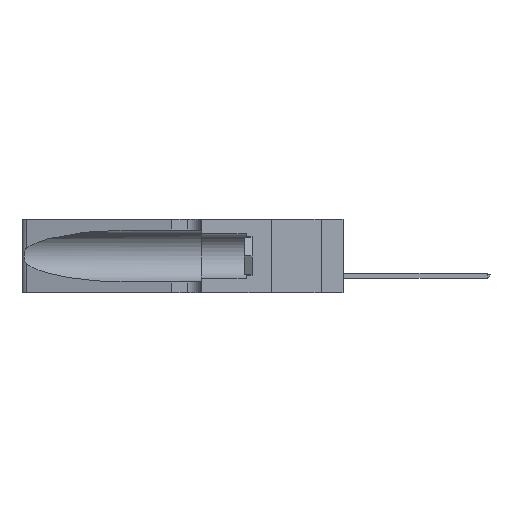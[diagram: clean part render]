
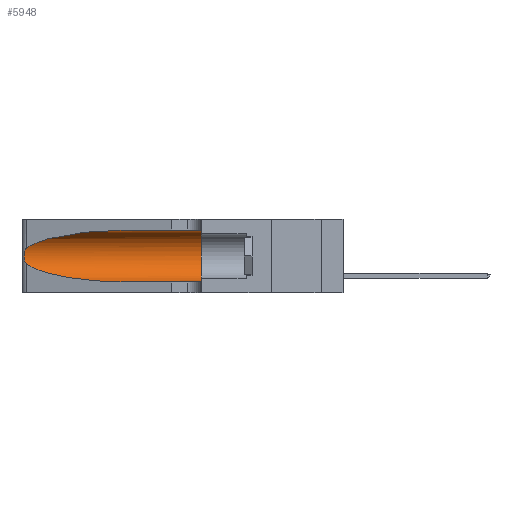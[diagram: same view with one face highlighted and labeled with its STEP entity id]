
A CAD part, left-side view. The second image highlights one B-rep face of the part: STEP entity #5948.
In plain terms, the highlighted cylindrical face has radius 3.308 mm (diameter 6.617 mm), a partial arc.
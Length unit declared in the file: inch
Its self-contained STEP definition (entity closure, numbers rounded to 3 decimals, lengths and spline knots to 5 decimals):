
#655 = CARTESIAN_POINT ( 'NONE',  ( 0.25555, 1.22993, 0.14849 ) ) ;
#1748 = LINE ( 'NONE', #39697, #17648 ) ;
#3922 = ORIENTED_EDGE ( 'NONE', *, *, #5991, .F. ) ;
#4035 = VECTOR ( 'NONE', #27838, 39.37008 ) ;
#4862 = CARTESIAN_POINT ( 'NONE',  ( 0.1305, 1.61858, 0.05475 ) ) ;
#5517 = EDGE_CURVE ( 'NONE', #15986, #20509, #34708, .T. ) ;
#5948 = ADVANCED_FACE ( 'NONE', ( #23339 ), #35680, .F. ) ;
#5991 = EDGE_CURVE ( 'NONE', #20962, #15986, #1748, .T. ) ;
#6048 = CARTESIAN_POINT ( 'NONE',  ( 0.1305, 0.35, 0.185 ) ) ;
#6563 = CARTESIAN_POINT ( 'NONE',  ( 0.26018, 1.23835, 0.19895 ) ) ;
#6578 = VERTEX_POINT ( 'NONE', #8494 ) ;
#6843 = CARTESIAN_POINT ( 'NONE',  ( 0.25487, 1.22718, 0.14631 ) ) ;
#7131 = CARTESIAN_POINT ( 'NONE',  ( 0.25639, 1.23186, 0.15144 ) ) ;
#7521 = AXIS2_PLACEMENT_3D ( 'NONE', #28760, #9085, #19129 ) ;
#8494 = CARTESIAN_POINT ( 'NONE',  ( 0.25487, 1.22718, 0.22369 ) ) ;
#9085 = DIRECTION ( 'NONE',  ( 0., -1., 0. ) ) ;
#9271 = CARTESIAN_POINT ( 'NONE',  ( 0.26075, 1.23896, 0.19203 ) ) ;
#9691 = CARTESIAN_POINT ( 'NONE',  ( 0.25789, 1.23486, 0.15765 ) ) ;
#9707 = VERTEX_POINT ( 'NONE', #18508 ) ;
#10004 = CARTESIAN_POINT ( 'NONE',  ( 0.1305, 0.72297, 0.31525 ) ) ;
#10328 = EDGE_CURVE ( 'NONE', #6578, #23851, #29841, .T. ) ;
#11489 = ORIENTED_EDGE ( 'NONE', *, *, #18581, .T. ) ;
#11865 = CARTESIAN_POINT ( 'NONE',  ( 0.18966, 0.96281, 0.05475 ) ) ;
#13286 = CARTESIAN_POINT ( 'NONE',  ( 0.18966, 0.96281, 0.31525 ) ) ;
#14525 =( BOUNDED_CURVE ( )  B_SPLINE_CURVE ( 3, ( #10004, #13286, #26381, #36300 ),
 .UNSPECIFIED., .F., .T. ) 
 B_SPLINE_CURVE_WITH_KNOTS ( ( 4, 4 ),
 ( 1.5708, 2.84003 ),
 .UNSPECIFIED. ) 
 CURVE ( )  GEOMETRIC_REPRESENTATION_ITEM ( )  RATIONAL_B_SPLINE_CURVE ( ( 1., 0.87, 0.87, 1. ) ) 
 REPRESENTATION_ITEM ( '' )  );
#15850 = CARTESIAN_POINT ( 'NONE',  ( 0.26075, 1.23896, 0.178 ) ) ;
#15986 = VERTEX_POINT ( 'NONE', #32086 ) ;
#17013 = ORIENTED_EDGE ( 'NONE', *, *, #5517, .F. ) ;
#17648 = VECTOR ( 'NONE', #29626, 39.37008 ) ;
#18508 = CARTESIAN_POINT ( 'NONE',  ( 0.1305, 0.72297, 0.05475 ) ) ;
#18581 = EDGE_CURVE ( 'NONE', #9707, #20509, #19427, .T. ) ;
#18585 = CARTESIAN_POINT ( 'NONE',  ( 0.25487, 1.22718, 0.22369 ) ) ;
#18779 = CARTESIAN_POINT ( 'NONE',  ( 0.1305, 0.35, 0.05475 ) ) ;
#19129 = DIRECTION ( 'NONE',  ( 0., 0., -1. ) ) ;
#19427 = LINE ( 'NONE', #4862, #4035 ) ;
#20509 = VERTEX_POINT ( 'NONE', #18779 ) ;
#20924 = ORIENTED_EDGE ( 'NONE', *, *, #25940, .T. ) ;
#20962 = VERTEX_POINT ( 'NONE', #34828 ) ;
#22037 = CARTESIAN_POINT ( 'NONE',  ( 0.25787, 1.23484, 0.2124 ) ) ;
#22477 = CARTESIAN_POINT ( 'NONE',  ( 0.26017, 1.23833, 0.17102 ) ) ;
#22758 = CARTESIAN_POINT ( 'NONE',  ( 0.25856, 1.23593, 0.16098 ) ) ;
#23339 = FACE_OUTER_BOUND ( 'NONE', #27698, .T. ) ;
#23851 = VERTEX_POINT ( 'NONE', #37448 ) ;
#25346 = CARTESIAN_POINT ( 'NONE',  ( 0.25854, 1.2359, 0.20912 ) ) ;
#25940 = EDGE_CURVE ( 'NONE', #23851, #9707, #38251, .T. ) ;
#26177 = EDGE_CURVE ( 'NONE', #20962, #6578, #14525, .T. ) ;
#26381 = CARTESIAN_POINT ( 'NONE',  ( 0.2373, 1.15595, 0.28018 ) ) ;
#26403 = DIRECTION ( 'NONE',  ( 0., 0., 1. ) ) ;
#26969 = DIRECTION ( 'NONE',  ( 0., 1., 0. ) ) ;
#27698 = EDGE_LOOP ( 'NONE', ( #40674, #36368, #20924, #11489, #17013, #3922 ) ) ;
#27838 = DIRECTION ( 'NONE',  ( 0., -1., 0. ) ) ;
#28095 = CARTESIAN_POINT ( 'NONE',  ( 0.25487, 1.22718, 0.14631 ) ) ;
#28219 = CARTESIAN_POINT ( 'NONE',  ( 0.25555, 1.22994, 0.2215 ) ) ;
#28760 = CARTESIAN_POINT ( 'NONE',  ( 0.1305, 1.61858, 0.185 ) ) ;
#29626 = DIRECTION ( 'NONE',  ( 0., -1., 0. ) ) ;
#29841 = B_SPLINE_CURVE_WITH_KNOTS ( 'NONE', 3,
 ( #18585, #28219, #38294, #22037, #25346, #6563, #9271, #15850, #22477, #22758, #9691, #7131, #655, #6843 ),
 .UNSPECIFIED., .F., .F.,
 ( 4, 2, 2, 2, 2, 2, 4 ),
 ( 0., 0.00027, 0.00053, 0.00107, 0.0016, 0.00187, 0.00214 ),
 .UNSPECIFIED. ) ;
#31265 = CARTESIAN_POINT ( 'NONE',  ( 0.1305, 0.72297, 0.05475 ) ) ;
#31683 = CARTESIAN_POINT ( 'NONE',  ( 0.2373, 1.15595, 0.08982 ) ) ;
#32086 = CARTESIAN_POINT ( 'NONE',  ( 0.1305, 0.35, 0.31525 ) ) ;
#34708 = CIRCLE ( 'NONE', #40789, 0.13025 ) ;
#34828 = CARTESIAN_POINT ( 'NONE',  ( 0.1305, 0.72297, 0.31525 ) ) ;
#35680 = CYLINDRICAL_SURFACE ( 'NONE', #7521, 0.13025 ) ;
#36300 = CARTESIAN_POINT ( 'NONE',  ( 0.25487, 1.22718, 0.22369 ) ) ;
#36368 = ORIENTED_EDGE ( 'NONE', *, *, #10328, .T. ) ;
#37448 = CARTESIAN_POINT ( 'NONE',  ( 0.25487, 1.22718, 0.14631 ) ) ;
#38251 =( BOUNDED_CURVE ( )  B_SPLINE_CURVE ( 3, ( #28095, #31683, #11865, #31265 ),
 .UNSPECIFIED., .F., .F. ) 
 B_SPLINE_CURVE_WITH_KNOTS ( ( 4, 4 ),
 ( 3.44316, 4.71239 ),
 .UNSPECIFIED. ) 
 CURVE ( )  GEOMETRIC_REPRESENTATION_ITEM ( )  RATIONAL_B_SPLINE_CURVE ( ( 1., 0.87, 0.87, 1. ) ) 
 REPRESENTATION_ITEM ( '' )  );
#38294 = CARTESIAN_POINT ( 'NONE',  ( 0.25639, 1.23184, 0.21858 ) ) ;
#39697 = CARTESIAN_POINT ( 'NONE',  ( 0.1305, 1.61858, 0.31525 ) ) ;
#40674 = ORIENTED_EDGE ( 'NONE', *, *, #26177, .T. ) ;
#40789 = AXIS2_PLACEMENT_3D ( 'NONE', #6048, #26969, #26403 ) ;
